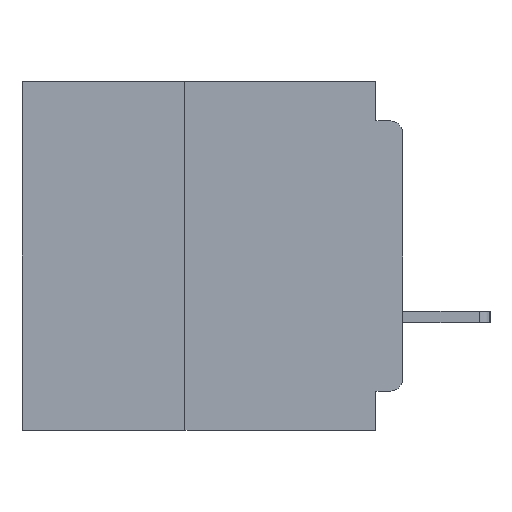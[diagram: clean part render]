
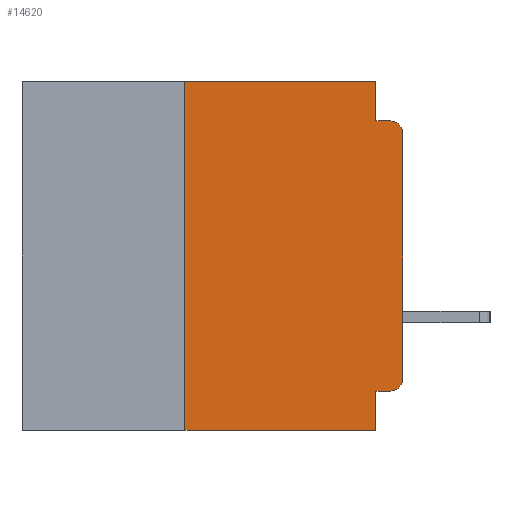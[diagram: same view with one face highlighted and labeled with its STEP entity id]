
A CAD part, left-side view. The second image highlights one B-rep face of the part: STEP entity #14620.
In plain terms, the highlighted planar face has unit normal (-1, 0, 0).
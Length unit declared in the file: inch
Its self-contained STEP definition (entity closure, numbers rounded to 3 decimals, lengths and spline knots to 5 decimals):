
#1260 = VECTOR ( 'NONE', #1534, 39.37008 ) ;
#1534 = DIRECTION ( 'NONE',  ( 0., -1., 0. ) ) ;
#3215 = ORIENTED_EDGE ( 'NONE', *, *, #14606, .T. ) ;
#3234 = ORIENTED_EDGE ( 'NONE', *, *, #22157, .F. ) ;
#3645 = CIRCLE ( 'NONE', #54084, 0.015 ) ;
#3889 = ORIENTED_EDGE ( 'NONE', *, *, #40266, .F. ) ;
#3995 = ORIENTED_EDGE ( 'NONE', *, *, #48370, .T. ) ;
#4266 = EDGE_CURVE ( 'NONE', #16501, #44039, #36776, .T. ) ;
#5725 = VECTOR ( 'NONE', #58309, 39.37008 ) ;
#5858 = DIRECTION ( 'NONE',  ( 0., 0., -1. ) ) ;
#6824 = ORIENTED_EDGE ( 'NONE', *, *, #47762, .F. ) ;
#6879 = EDGE_CURVE ( 'NONE', #33231, #12969, #16233, .T. ) ;
#8410 = PLANE ( 'NONE',  #34128 ) ;
#9766 = ORIENTED_EDGE ( 'NONE', *, *, #6879, .F. ) ;
#10922 = VERTEX_POINT ( 'NONE', #33190 ) ;
#11234 = ORIENTED_EDGE ( 'NONE', *, *, #16219, .F. ) ;
#12969 = VERTEX_POINT ( 'NONE', #50701 ) ;
#14330 = LINE ( 'NONE', #20168, #25256 ) ;
#14606 = EDGE_CURVE ( 'NONE', #25912, #54716, #52903, .T. ) ;
#14620 = ADVANCED_FACE ( 'NONE', ( #39347 ), #8410, .F. ) ;
#14761 = VECTOR ( 'NONE', #48273, 39.37008 ) ;
#15259 = LINE ( 'NONE', #43348, #1260 ) ;
#15409 = CARTESIAN_POINT ( 'NONE',  ( 0., 0.015, -0.34 ) ) ;
#15481 = LINE ( 'NONE', #17598, #49279 ) ;
#16219 = EDGE_CURVE ( 'NONE', #35452, #33231, #15259, .T. ) ;
#16233 = LINE ( 'NONE', #20769, #14761 ) ;
#16501 = VERTEX_POINT ( 'NONE', #31306 ) ;
#17598 = CARTESIAN_POINT ( 'NONE',  ( 0., 0.25, -0.4 ) ) ;
#17783 = ORIENTED_EDGE ( 'NONE', *, *, #34701, .T. ) ;
#17785 = DIRECTION ( 'NONE',  ( 0., 0., -1. ) ) ;
#18176 = LINE ( 'NONE', #49107, #5725 ) ;
#18235 = CARTESIAN_POINT ( 'NONE',  ( 0., 0.015, -0.06 ) ) ;
#20096 = DIRECTION ( 'NONE',  ( 0., 0., -1. ) ) ;
#20168 = CARTESIAN_POINT ( 'NONE',  ( 0., 0., -0.045 ) ) ;
#20769 = CARTESIAN_POINT ( 'NONE',  ( 0., 0.031, 0. ) ) ;
#21809 = CARTESIAN_POINT ( 'NONE',  ( 0., 0., -0.06 ) ) ;
#21896 = CARTESIAN_POINT ( 'NONE',  ( 0., 0., 0. ) ) ;
#22157 = EDGE_CURVE ( 'NONE', #10922, #54716, #32594, .T. ) ;
#22478 = DIRECTION ( 'NONE',  ( 0., 0., 1. ) ) ;
#22932 = DIRECTION ( 'NONE',  ( 0., 0., -1. ) ) ;
#25256 = VECTOR ( 'NONE', #56851, 39.37008 ) ;
#25912 = VERTEX_POINT ( 'NONE', #39316 ) ;
#26594 = DIRECTION ( 'NONE',  ( 0., 0., 1. ) ) ;
#28049 = EDGE_CURVE ( 'NONE', #25912, #35452, #15481, .T. ) ;
#31306 = CARTESIAN_POINT ( 'NONE',  ( 0., 0., -0.34 ) ) ;
#31554 = DIRECTION ( 'NONE',  ( 0., -1., 0. ) ) ;
#32594 = LINE ( 'NONE', #56457, #43343 ) ;
#33190 = CARTESIAN_POINT ( 'NONE',  ( 0., 0.031, -0.355 ) ) ;
#33231 = VERTEX_POINT ( 'NONE', #43986 ) ;
#34128 = AXIS2_PLACEMENT_3D ( 'NONE', #40774, #45369, #17785 ) ;
#34701 = EDGE_CURVE ( 'NONE', #44039, #56933, #3645, .T. ) ;
#35452 = VERTEX_POINT ( 'NONE', #54779 ) ;
#36739 = EDGE_LOOP ( 'NONE', ( #52241, #17783, #6824, #9766, #11234, #53713, #3215, #3234, #3889, #3995 ) ) ;
#36776 = LINE ( 'NONE', #21896, #59650 ) ;
#39316 = CARTESIAN_POINT ( 'NONE',  ( 0., 0.25, -0.4 ) ) ;
#39347 = FACE_OUTER_BOUND ( 'NONE', #36739, .T. ) ;
#40266 = EDGE_CURVE ( 'NONE', #42259, #10922, #18176, .T. ) ;
#40774 = CARTESIAN_POINT ( 'NONE',  ( 0., 0.437, 0. ) ) ;
#40973 = CIRCLE ( 'NONE', #50838, 0.015 ) ;
#42259 = VERTEX_POINT ( 'NONE', #56545 ) ;
#43343 = VECTOR ( 'NONE', #5858, 39.37008 ) ;
#43348 = CARTESIAN_POINT ( 'NONE',  ( 0., 0.437, 0. ) ) ;
#43986 = CARTESIAN_POINT ( 'NONE',  ( 0., 0.031, 0. ) ) ;
#44039 = VERTEX_POINT ( 'NONE', #21809 ) ;
#45369 = DIRECTION ( 'NONE',  ( 1., 0., 0. ) ) ;
#47597 = DIRECTION ( 'NONE',  ( -1., 0., 0. ) ) ;
#47762 = EDGE_CURVE ( 'NONE', #12969, #56933, #14330, .T. ) ;
#48273 = DIRECTION ( 'NONE',  ( 0., 0., -1. ) ) ;
#48370 = EDGE_CURVE ( 'NONE', #42259, #16501, #40973, .T. ) ;
#49107 = CARTESIAN_POINT ( 'NONE',  ( 0., 0., -0.355 ) ) ;
#49279 = VECTOR ( 'NONE', #22478, 39.37008 ) ;
#50378 = DIRECTION ( 'NONE',  ( -1., 0., 0. ) ) ;
#50701 = CARTESIAN_POINT ( 'NONE',  ( 0., 0.031, -0.045 ) ) ;
#50789 = CARTESIAN_POINT ( 'NONE',  ( 0., 0.031, -0.4 ) ) ;
#50838 = AXIS2_PLACEMENT_3D ( 'NONE', #15409, #47597, #20096 ) ;
#51476 = VECTOR ( 'NONE', #31554, 39.37008 ) ;
#52241 = ORIENTED_EDGE ( 'NONE', *, *, #4266, .T. ) ;
#52903 = LINE ( 'NONE', #54301, #51476 ) ;
#53713 = ORIENTED_EDGE ( 'NONE', *, *, #28049, .F. ) ;
#54084 = AXIS2_PLACEMENT_3D ( 'NONE', #18235, #50378, #22932 ) ;
#54301 = CARTESIAN_POINT ( 'NONE',  ( 0., 0.437, -0.4 ) ) ;
#54716 = VERTEX_POINT ( 'NONE', #50789 ) ;
#54779 = CARTESIAN_POINT ( 'NONE',  ( 0., 0.25, 0. ) ) ;
#56457 = CARTESIAN_POINT ( 'NONE',  ( 0., 0.031, -0.4 ) ) ;
#56545 = CARTESIAN_POINT ( 'NONE',  ( 0., 0.015, -0.355 ) ) ;
#56851 = DIRECTION ( 'NONE',  ( 0., -1., 0. ) ) ;
#56933 = VERTEX_POINT ( 'NONE', #58546 ) ;
#58309 = DIRECTION ( 'NONE',  ( 0., 1., 0. ) ) ;
#58546 = CARTESIAN_POINT ( 'NONE',  ( 0., 0.015, -0.045 ) ) ;
#59650 = VECTOR ( 'NONE', #26594, 39.37008 ) ;
